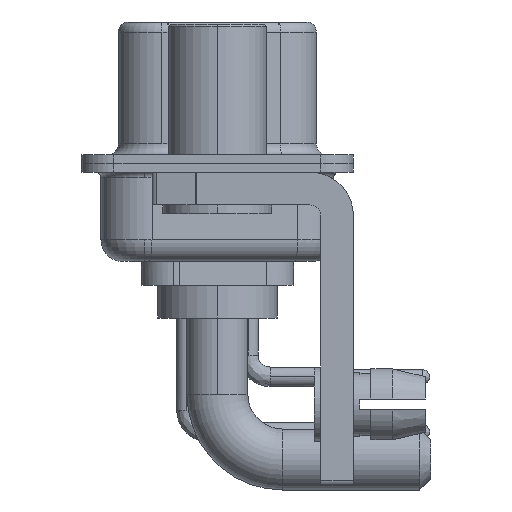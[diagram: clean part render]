
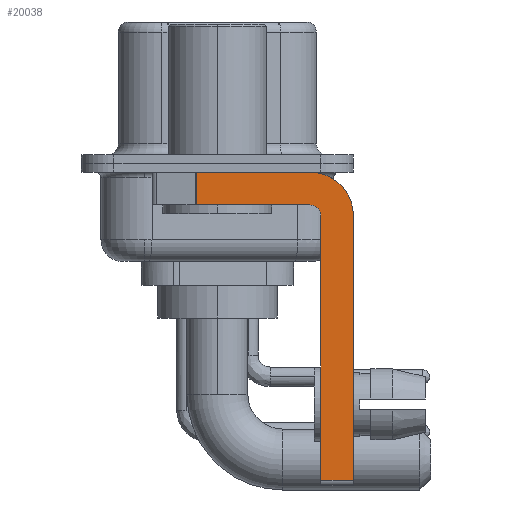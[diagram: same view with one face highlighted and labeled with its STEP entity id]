
A CAD part, left-side view. The second image highlights one B-rep face of the part: STEP entity #20038.
In plain terms, the highlighted planar face has unit normal (-1, 0, 0).
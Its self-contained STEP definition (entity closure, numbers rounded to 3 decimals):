
#808 = CIRCLE ( 'NONE', #16207, 2. ) ;
#1343 = CARTESIAN_POINT ( 'NONE',  ( -2.9, 0.978, -0.4 ) ) ;
#1622 = DIRECTION ( 'NONE',  ( 0., 1., 0. ) ) ;
#3011 = ORIENTED_EDGE ( 'NONE', *, *, #3038, .T. ) ;
#3038 = EDGE_CURVE ( 'NONE', #19844, #6671, #25911, .T. ) ;
#3746 = CARTESIAN_POINT ( 'NONE',  ( -2.9, -4.25, -1.9 ) ) ;
#4516 = DIRECTION ( 'NONE',  ( 0., 0., -1. ) ) ;
#4545 = ORIENTED_EDGE ( 'NONE', *, *, #14081, .F. ) ;
#4999 = CIRCLE ( 'NONE', #10881, 0.5 ) ;
#5462 = VECTOR ( 'NONE', #19326, 1000. ) ;
#5630 = VECTOR ( 'NONE', #4516, 1000. ) ;
#5665 = CARTESIAN_POINT ( 'NONE',  ( -2.9, -6.25, -2.4 ) ) ;
#5670 = VERTEX_POINT ( 'NONE', #10803 ) ;
#5730 = CARTESIAN_POINT ( 'NONE',  ( -2.9, -4.25, -2.4 ) ) ;
#6147 = LINE ( 'NONE', #3746, #15068 ) ;
#6223 = EDGE_CURVE ( 'NONE', #11045, #21285, #4999, .T. ) ;
#6671 = VERTEX_POINT ( 'NONE', #26187 ) ;
#6844 = CARTESIAN_POINT ( 'NONE',  ( -2.9, -4.25, -1.9 ) ) ;
#6913 = ORIENTED_EDGE ( 'NONE', *, *, #20148, .F. ) ;
#7548 = DIRECTION ( 'NONE',  ( 1., 0., 0. ) ) ;
#7696 = DIRECTION ( 'NONE',  ( 0., -1., 0. ) ) ;
#7747 = VERTEX_POINT ( 'NONE', #5665 ) ;
#7852 = FACE_OUTER_BOUND ( 'NONE', #11084, .T. ) ;
#8741 = CARTESIAN_POINT ( 'NONE',  ( -2.9, 0.978, -1.9 ) ) ;
#8746 = ORIENTED_EDGE ( 'NONE', *, *, #12935, .F. ) ;
#9085 = CARTESIAN_POINT ( 'NONE',  ( -2.9, 3., -0.4 ) ) ;
#9781 = VERTEX_POINT ( 'NONE', #12923 ) ;
#9844 = EDGE_CURVE ( 'NONE', #5670, #11045, #10377, .T. ) ;
#10377 = LINE ( 'NONE', #12502, #15124 ) ;
#10803 = CARTESIAN_POINT ( 'NONE',  ( -2.9, -4.75, -14.55 ) ) ;
#10881 = AXIS2_PLACEMENT_3D ( 'NONE', #24111, #13457, #19709 ) ;
#11045 = VERTEX_POINT ( 'NONE', #19036 ) ;
#11084 = EDGE_LOOP ( 'NONE', ( #6913, #3011, #26801, #13479, #23157, #22589, #8746, #4545 ) ) ;
#12502 = CARTESIAN_POINT ( 'NONE',  ( -2.9, -4.75, -14.8 ) ) ;
#12923 = CARTESIAN_POINT ( 'NONE',  ( -2.9, -6.25, -14.55 ) ) ;
#12935 = EDGE_CURVE ( 'NONE', #7747, #9781, #14855, .T. ) ;
#13457 = DIRECTION ( 'NONE',  ( -1., 0., 0. ) ) ;
#13479 = ORIENTED_EDGE ( 'NONE', *, *, #6223, .F. ) ;
#14081 = EDGE_CURVE ( 'NONE', #24015, #7747, #808, .T. ) ;
#14393 = VECTOR ( 'NONE', #7696, 1000. ) ;
#14855 = LINE ( 'NONE', #19107, #25660 ) ;
#15068 = VECTOR ( 'NONE', #1622, 1000. ) ;
#15124 = VECTOR ( 'NONE', #27680, 1000. ) ;
#15206 = DIRECTION ( 'NONE',  ( 0., 0., -1. ) ) ;
#15379 = EDGE_CURVE ( 'NONE', #5670, #9781, #18175, .T. ) ;
#15778 = DIRECTION ( 'NONE',  ( 0., 0., -1. ) ) ;
#16207 = AXIS2_PLACEMENT_3D ( 'NONE', #26964, #7548, #15778 ) ;
#16799 = AXIS2_PLACEMENT_3D ( 'NONE', #5730, #25839, #15206 ) ;
#17586 = CARTESIAN_POINT ( 'NONE',  ( -2.9, -4.25, -0.4 ) ) ;
#18175 = LINE ( 'NONE', #20593, #14393 ) ;
#19036 = CARTESIAN_POINT ( 'NONE',  ( -2.9, -4.75, -2.4 ) ) ;
#19107 = CARTESIAN_POINT ( 'NONE',  ( -2.9, -6.25, -2.4 ) ) ;
#19326 = DIRECTION ( 'NONE',  ( 0., -1., 0. ) ) ;
#19709 = DIRECTION ( 'NONE',  ( 0., 0., 1. ) ) ;
#19844 = VERTEX_POINT ( 'NONE', #1343 ) ;
#19871 = LINE ( 'NONE', #9085, #5462 ) ;
#20038 = ADVANCED_FACE ( 'NONE', ( #7852 ), #25164, .F. ) ;
#20148 = EDGE_CURVE ( 'NONE', #19844, #24015, #19871, .T. ) ;
#20593 = CARTESIAN_POINT ( 'NONE',  ( -2.9, -4.25, -14.55 ) ) ;
#21285 = VERTEX_POINT ( 'NONE', #6844 ) ;
#22530 = EDGE_CURVE ( 'NONE', #21285, #6671, #6147, .T. ) ;
#22589 = ORIENTED_EDGE ( 'NONE', *, *, #15379, .T. ) ;
#23157 = ORIENTED_EDGE ( 'NONE', *, *, #9844, .F. ) ;
#24015 = VERTEX_POINT ( 'NONE', #17586 ) ;
#24111 = CARTESIAN_POINT ( 'NONE',  ( -2.9, -4.25, -2.4 ) ) ;
#25164 = PLANE ( 'NONE',  #16799 ) ;
#25362 = DIRECTION ( 'NONE',  ( 0., 0., -1. ) ) ;
#25660 = VECTOR ( 'NONE', #25362, 1000. ) ;
#25839 = DIRECTION ( 'NONE',  ( 1., 0., 0. ) ) ;
#25911 = LINE ( 'NONE', #8741, #5630 ) ;
#26187 = CARTESIAN_POINT ( 'NONE',  ( -2.9, 0.978, -1.9 ) ) ;
#26801 = ORIENTED_EDGE ( 'NONE', *, *, #22530, .F. ) ;
#26964 = CARTESIAN_POINT ( 'NONE',  ( -2.9, -4.25, -2.4 ) ) ;
#27680 = DIRECTION ( 'NONE',  ( 0., 0., 1. ) ) ;
